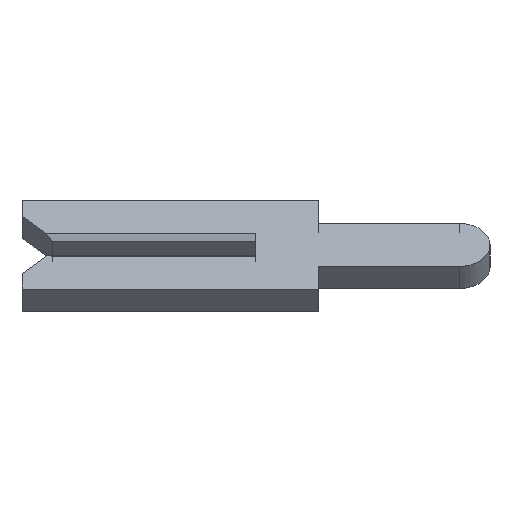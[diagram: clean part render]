
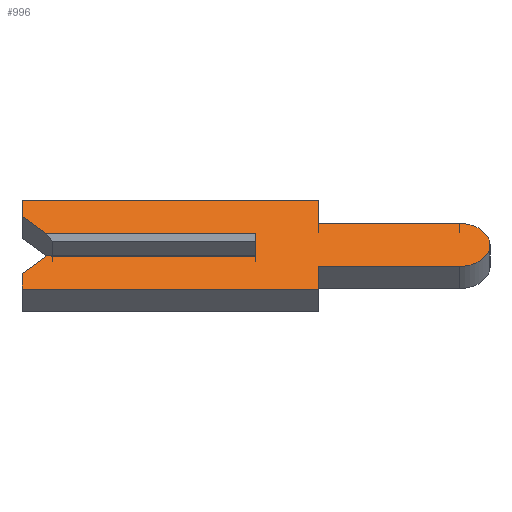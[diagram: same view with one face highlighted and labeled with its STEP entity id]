
A CAD part, left-side view. The second image highlights one B-rep face of the part: STEP entity #996.
In plain terms, the highlighted face is planar.
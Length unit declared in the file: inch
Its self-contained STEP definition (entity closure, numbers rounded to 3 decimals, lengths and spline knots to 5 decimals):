
#30 = CARTESIAN_POINT ( 'NONE',  ( -0.01, 0.15, -0.04 ) ) ;
#63 = CARTESIAN_POINT ( 'NONE',  ( -0.01, 0.1305, 0.0065 ) ) ;
#69 = CARTESIAN_POINT ( 'NONE',  ( -0.01, -0.1305, 0. ) ) ;
#75 = ORIENTED_EDGE ( 'NONE', *, *, #1287, .F. ) ;
#89 = CARTESIAN_POINT ( 'NONE',  ( -0.01, -0.04, 0.0195 ) ) ;
#92 = LINE ( 'NONE', #657, #422 ) ;
#93 = LINE ( 'NONE', #140, #764 ) ;
#115 = DIRECTION ( 'NONE',  ( 0., -1., 0. ) ) ;
#140 = CARTESIAN_POINT ( 'NONE',  ( -0.01, -0.1305, -0.01 ) ) ;
#145 = EDGE_CURVE ( 'NONE', #890, #1777, #971, .T. ) ;
#169 = CARTESIAN_POINT ( 'NONE',  ( -0.01, -0.04, -0.0195 ) ) ;
#196 = VERTEX_POINT ( 'NONE', #651 ) ;
#222 = VERTEX_POINT ( 'NONE', #1069 ) ;
#234 = DIRECTION ( 'NONE',  ( 0., -0.707, 0.707 ) ) ;
#239 = EDGE_CURVE ( 'NONE', #1299, #515, #388, .T. ) ;
#261 = EDGE_CURVE ( 'NONE', #222, #1385, #1232, .T. ) ;
#280 = DIRECTION ( 'NONE',  ( 0., 0., 1. ) ) ;
#281 = VERTEX_POINT ( 'NONE', #1320 ) ;
#299 = CARTESIAN_POINT ( 'NONE',  ( -0.01, -0.04, -0.04 ) ) ;
#300 = LINE ( 'NONE', #837, #1436 ) ;
#306 = CARTESIAN_POINT ( 'NONE',  ( -0.01, -0.04, 0.0195 ) ) ;
#328 = EDGE_CURVE ( 'NONE', #688, #196, #1570, .T. ) ;
#342 = DIRECTION ( 'NONE',  ( 0., -1., 0. ) ) ;
#347 = VERTEX_POINT ( 'NONE', #1490 ) ;
#349 = ORIENTED_EDGE ( 'NONE', *, *, #1580, .F. ) ;
#354 = CARTESIAN_POINT ( 'NONE',  ( -0.01, 0.15, 0.01 ) ) ;
#372 = CARTESIAN_POINT ( 'NONE',  ( -0.01, 0.15, -0.04 ) ) ;
#388 = LINE ( 'NONE', #372, #664 ) ;
#389 = CARTESIAN_POINT ( 'NONE',  ( -0.01, -0.1305, 0.0195 ) ) ;
#402 = VECTOR ( 'NONE', #115, 39.37008 ) ;
#422 = VECTOR ( 'NONE', #1637, 39.37008 ) ;
#430 = ORIENTED_EDGE ( 'NONE', *, *, #145, .F. ) ;
#442 = EDGE_CURVE ( 'NONE', #196, #281, #93, .T. ) ;
#453 = VECTOR ( 'NONE', #577, 39.37008 ) ;
#479 = CARTESIAN_POINT ( 'NONE',  ( -0.01, -0.04, -0.04 ) ) ;
#508 = EDGE_CURVE ( 'NONE', #847, #890, #1460, .T. ) ;
#515 = VERTEX_POINT ( 'NONE', #30 ) ;
#552 = EDGE_CURVE ( 'NONE', #281, #1423, #300, .T. ) ;
#568 = VECTOR ( 'NONE', #342, 39.37008 ) ;
#571 = VECTOR ( 'NONE', #234, 39.37008 ) ;
#572 = DIRECTION ( 'NONE',  ( 0., 0., -1. ) ) ;
#577 = DIRECTION ( 'NONE',  ( 0., 0.707, 0.707 ) ) ;
#593 = CARTESIAN_POINT ( 'NONE',  ( -0.01, 0.15, -0.026 ) ) ;
#602 = ORIENTED_EDGE ( 'NONE', *, *, #261, .F. ) ;
#618 = DIRECTION ( 'NONE',  ( 1., 0., 0. ) ) ;
#651 = CARTESIAN_POINT ( 'NONE',  ( -0.01, 0.134, -0.01 ) ) ;
#657 = CARTESIAN_POINT ( 'NONE',  ( -0.01, -0.04, -0.0195 ) ) ;
#664 = VECTOR ( 'NONE', #935, 39.37008 ) ;
#667 = ORIENTED_EDGE ( 'NONE', *, *, #239, .F. ) ;
#686 = VECTOR ( 'NONE', #572, 39.37008 ) ;
#688 = VERTEX_POINT ( 'NONE', #593 ) ;
#731 = EDGE_CURVE ( 'NONE', #347, #222, #949, .T. ) ;
#742 = VERTEX_POINT ( 'NONE', #169 ) ;
#747 = EDGE_CURVE ( 'NONE', #742, #1299, #868, .T. ) ;
#752 = CARTESIAN_POINT ( 'NONE',  ( -0.01, 0., 0.01 ) ) ;
#764 = VECTOR ( 'NONE', #1374, 39.37008 ) ;
#766 = ORIENTED_EDGE ( 'NONE', *, *, #442, .F. ) ;
#798 = CIRCLE ( 'NONE', #1500, 0.0195 ) ;
#799 = CARTESIAN_POINT ( 'NONE',  ( -0.01, 0.1305, -0.0065 ) ) ;
#837 = CARTESIAN_POINT ( 'NONE',  ( -0.01, 0., 0.0065 ) ) ;
#845 = VERTEX_POINT ( 'NONE', #1705 ) ;
#847 = VERTEX_POINT ( 'NONE', #1426 ) ;
#868 = LINE ( 'NONE', #299, #686 ) ;
#890 = VERTEX_POINT ( 'NONE', #306 ) ;
#910 = DIRECTION ( 'NONE',  ( 0., -1., 0. ) ) ;
#928 = VECTOR ( 'NONE', #1196, 39.37008 ) ;
#930 = ORIENTED_EDGE ( 'NONE', *, *, #1037, .T. ) ;
#935 = DIRECTION ( 'NONE',  ( 0., 1., 0. ) ) ;
#949 = LINE ( 'NONE', #63, #453 ) ;
#971 = LINE ( 'NONE', #89, #402 ) ;
#972 = DIRECTION ( 'NONE',  ( 0., 0., -1. ) ) ;
#993 = VECTOR ( 'NONE', #1767, 39.37008 ) ;
#996 = ADVANCED_FACE ( 'NONE', ( #1522 ), #1005, .F. ) ;
#1005 = PLANE ( 'NONE',  #1401 ) ;
#1037 = EDGE_CURVE ( 'NONE', #347, #1423, #1360, .T. ) ;
#1069 = CARTESIAN_POINT ( 'NONE',  ( -0.01, 0.15, 0.026 ) ) ;
#1131 = ORIENTED_EDGE ( 'NONE', *, *, #552, .F. ) ;
#1165 = CARTESIAN_POINT ( 'NONE',  ( -0.01, 0.15, 0.04 ) ) ;
#1171 = VECTOR ( 'NONE', #910, 39.37008 ) ;
#1175 = ORIENTED_EDGE ( 'NONE', *, *, #1528, .F. ) ;
#1196 = DIRECTION ( 'NONE',  ( 0., 0., 1. ) ) ;
#1231 = LINE ( 'NONE', #1624, #993 ) ;
#1232 = LINE ( 'NONE', #1771, #928 ) ;
#1287 = EDGE_CURVE ( 'NONE', #1777, #845, #798, .T. ) ;
#1299 = VERTEX_POINT ( 'NONE', #479 ) ;
#1300 = ORIENTED_EDGE ( 'NONE', *, *, #731, .F. ) ;
#1305 = CARTESIAN_POINT ( 'NONE',  ( -0.01, -0.1305, 0. ) ) ;
#1310 = DIRECTION ( 'NONE',  ( 1., 0., 0. ) ) ;
#1320 = CARTESIAN_POINT ( 'NONE',  ( -0.01, 0., -0.01 ) ) ;
#1360 = LINE ( 'NONE', #354, #568 ) ;
#1366 = ORIENTED_EDGE ( 'NONE', *, *, #747, .F. ) ;
#1374 = DIRECTION ( 'NONE',  ( 0., -1., 0. ) ) ;
#1379 = EDGE_CURVE ( 'NONE', #1385, #847, #1704, .T. ) ;
#1382 = CARTESIAN_POINT ( 'NONE',  ( -0.01, -0.04, 0.04 ) ) ;
#1385 = VERTEX_POINT ( 'NONE', #1165 ) ;
#1401 = AXIS2_PLACEMENT_3D ( 'NONE', #69, #1310, #1450 ) ;
#1423 = VERTEX_POINT ( 'NONE', #752 ) ;
#1426 = CARTESIAN_POINT ( 'NONE',  ( -0.01, -0.04, 0.04 ) ) ;
#1436 = VECTOR ( 'NONE', #280, 39.37008 ) ;
#1443 = EDGE_LOOP ( 'NONE', ( #930, #1131, #766, #1688, #1175, #667, #1366, #349, #75, #430, #1615, #1594, #602, #1300 ) ) ;
#1450 = DIRECTION ( 'NONE',  ( 0., 0., -1. ) ) ;
#1460 = LINE ( 'NONE', #1382, #1613 ) ;
#1490 = CARTESIAN_POINT ( 'NONE',  ( -0.01, 0.134, 0.01 ) ) ;
#1500 = AXIS2_PLACEMENT_3D ( 'NONE', #1305, #618, #1744 ) ;
#1522 = FACE_OUTER_BOUND ( 'NONE', #1443, .T. ) ;
#1528 = EDGE_CURVE ( 'NONE', #515, #688, #1231, .T. ) ;
#1570 = LINE ( 'NONE', #799, #571 ) ;
#1580 = EDGE_CURVE ( 'NONE', #845, #742, #92, .T. ) ;
#1594 = ORIENTED_EDGE ( 'NONE', *, *, #1379, .F. ) ;
#1613 = VECTOR ( 'NONE', #972, 39.37008 ) ;
#1615 = ORIENTED_EDGE ( 'NONE', *, *, #508, .F. ) ;
#1624 = CARTESIAN_POINT ( 'NONE',  ( -0.01, 0.15, -0.026 ) ) ;
#1637 = DIRECTION ( 'NONE',  ( 0., 1., 0. ) ) ;
#1688 = ORIENTED_EDGE ( 'NONE', *, *, #328, .F. ) ;
#1704 = LINE ( 'NONE', #1760, #1171 ) ;
#1705 = CARTESIAN_POINT ( 'NONE',  ( -0.01, -0.1305, -0.0195 ) ) ;
#1744 = DIRECTION ( 'NONE',  ( 0., 0., -1. ) ) ;
#1760 = CARTESIAN_POINT ( 'NONE',  ( -0.01, 0.15, 0.04 ) ) ;
#1767 = DIRECTION ( 'NONE',  ( 0., 0., 1. ) ) ;
#1771 = CARTESIAN_POINT ( 'NONE',  ( -0.01, 0.15, 0.026 ) ) ;
#1777 = VERTEX_POINT ( 'NONE', #389 ) ;
